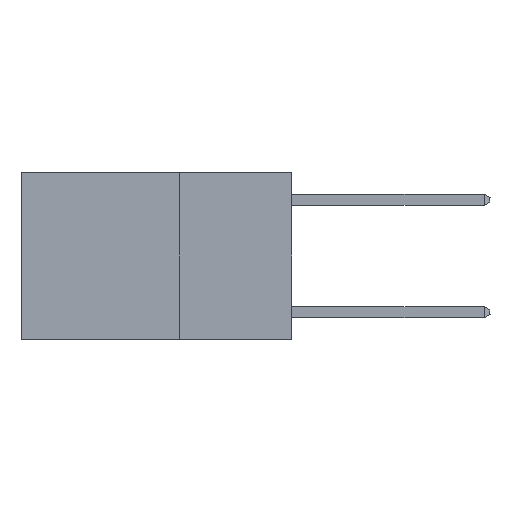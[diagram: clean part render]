
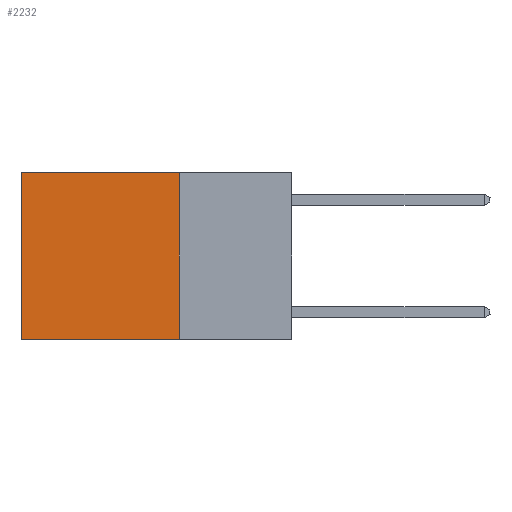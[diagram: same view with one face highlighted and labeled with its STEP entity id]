
A CAD part, left-side view. The second image highlights one B-rep face of the part: STEP entity #2232.
In plain terms, the highlighted planar face has unit normal (-1, 0, 0).
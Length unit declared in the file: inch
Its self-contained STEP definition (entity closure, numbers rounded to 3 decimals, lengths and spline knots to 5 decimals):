
#411 = CARTESIAN_POINT ( 'NONE',  ( 0.2625, 0.25, -0.37 ) ) ;
#640 = CARTESIAN_POINT ( 'NONE',  ( 0.2625, 0.25, 0. ) ) ;
#1112 = LINE ( 'NONE', #10183, #20365 ) ;
#1669 = CARTESIAN_POINT ( 'NONE',  ( 0.2625, 0.25, 0. ) ) ;
#2019 = EDGE_CURVE ( 'NONE', #2145, #17853, #5661, .T. ) ;
#2145 = VERTEX_POINT ( 'NONE', #2379 ) ;
#2232 = ADVANCED_FACE ( 'NONE', ( #6601 ), #17873, .F. ) ;
#2379 = CARTESIAN_POINT ( 'NONE',  ( 0.2625, 0.6, 0. ) ) ;
#2572 = DIRECTION ( 'NONE',  ( 0., 0., -1. ) ) ;
#3111 = DIRECTION ( 'NONE',  ( 0., 1., 0. ) ) ;
#3366 = LINE ( 'NONE', #1669, #7627 ) ;
#3652 = EDGE_CURVE ( 'NONE', #21520, #17853, #4685, .T. ) ;
#3849 = DIRECTION ( 'NONE',  ( 0., 0., -1. ) ) ;
#4685 = LINE ( 'NONE', #19728, #20637 ) ;
#5640 = CARTESIAN_POINT ( 'NONE',  ( 0.2625, 0.6, -0.37 ) ) ;
#5661 = LINE ( 'NONE', #20463, #17569 ) ;
#6601 = FACE_OUTER_BOUND ( 'NONE', #16773, .T. ) ;
#7409 = ORIENTED_EDGE ( 'NONE', *, *, #3652, .F. ) ;
#7627 = VECTOR ( 'NONE', #17061, 39.37008 ) ;
#8665 = DIRECTION ( 'NONE',  ( 1., 0., 0. ) ) ;
#9336 = EDGE_CURVE ( 'NONE', #13843, #21520, #1112, .T. ) ;
#10039 = EDGE_CURVE ( 'NONE', #13843, #2145, #3366, .T. ) ;
#10183 = CARTESIAN_POINT ( 'NONE',  ( 0.2625, 0.25, 0. ) ) ;
#11945 = DIRECTION ( 'NONE',  ( 0., 0., -1. ) ) ;
#13843 = VERTEX_POINT ( 'NONE', #640 ) ;
#16773 = EDGE_LOOP ( 'NONE', ( #21442, #7409, #22606, #22544 ) ) ;
#17061 = DIRECTION ( 'NONE',  ( 0., 1., 0. ) ) ;
#17569 = VECTOR ( 'NONE', #3849, 39.37008 ) ;
#17853 = VERTEX_POINT ( 'NONE', #5640 ) ;
#17873 = PLANE ( 'NONE',  #21102 ) ;
#19728 = CARTESIAN_POINT ( 'NONE',  ( 0.2625, 0.25, -0.37 ) ) ;
#20365 = VECTOR ( 'NONE', #2572, 39.37008 ) ;
#20463 = CARTESIAN_POINT ( 'NONE',  ( 0.2625, 0.6, 0. ) ) ;
#20637 = VECTOR ( 'NONE', #3111, 39.37008 ) ;
#21102 = AXIS2_PLACEMENT_3D ( 'NONE', #21306, #8665, #11945 ) ;
#21306 = CARTESIAN_POINT ( 'NONE',  ( 0.2625, 0.25, 0. ) ) ;
#21442 = ORIENTED_EDGE ( 'NONE', *, *, #2019, .T. ) ;
#21520 = VERTEX_POINT ( 'NONE', #411 ) ;
#22544 = ORIENTED_EDGE ( 'NONE', *, *, #10039, .T. ) ;
#22606 = ORIENTED_EDGE ( 'NONE', *, *, #9336, .F. ) ;
